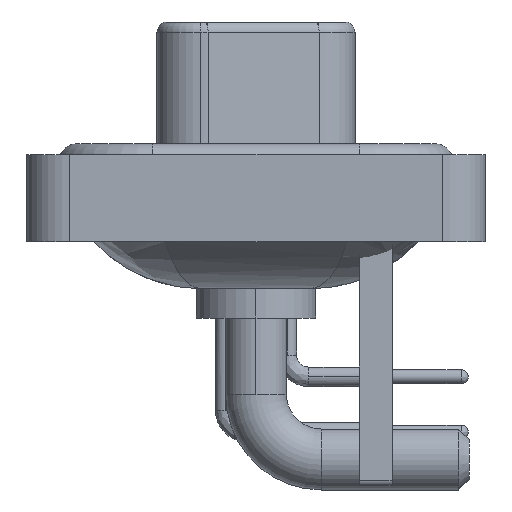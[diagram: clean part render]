
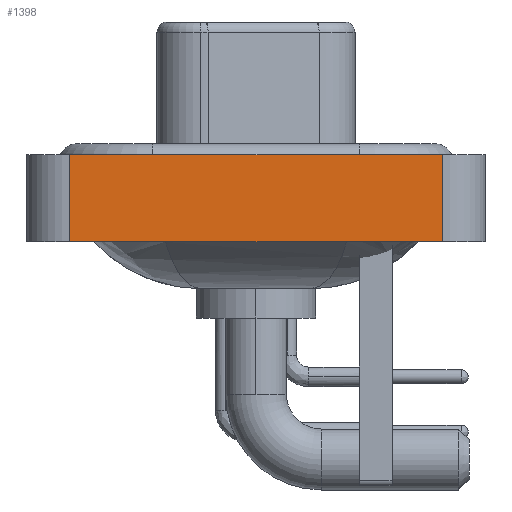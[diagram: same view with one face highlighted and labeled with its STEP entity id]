
A CAD part, left-side view. The second image highlights one B-rep face of the part: STEP entity #1398.
In plain terms, the highlighted planar face has unit normal (-1, 0, 0).
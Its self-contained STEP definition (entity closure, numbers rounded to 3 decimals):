
#428 = PLANE ( 'NONE',  #26858 ) ;
#519 = CARTESIAN_POINT ( 'NONE',  ( -7.35, 8.55, -3.6 ) ) ;
#929 = CARTESIAN_POINT ( 'NONE',  ( -7.35, 8.55, -3.6 ) ) ;
#1398 = ADVANCED_FACE ( 'NONE', ( #18277 ), #428, .T. ) ;
#2230 = EDGE_CURVE ( 'NONE', #17296, #16512, #19049, .T. ) ;
#3063 = DIRECTION ( 'NONE',  ( -1., 0., 0. ) ) ;
#4238 = CARTESIAN_POINT ( 'NONE',  ( -7.35, 8.55, 0.4 ) ) ;
#6524 = VECTOR ( 'NONE', #18590, 1000. ) ;
#7141 = VECTOR ( 'NONE', #9391, 1000. ) ;
#9391 = DIRECTION ( 'NONE',  ( 0., 0., 1. ) ) ;
#9456 = CARTESIAN_POINT ( 'NONE',  ( -7.35, -8.55, -3.6 ) ) ;
#9499 = LINE ( 'NONE', #13789, #28055 ) ;
#9691 = CARTESIAN_POINT ( 'NONE',  ( -7.35, -8.55, 0.4 ) ) ;
#10008 = EDGE_LOOP ( 'NONE', ( #10901, #12524, #17019, #13452 ) ) ;
#10021 = CARTESIAN_POINT ( 'NONE',  ( -7.35, -8.55, -3.6 ) ) ;
#10263 = EDGE_CURVE ( 'NONE', #16512, #11196, #16607, .T. ) ;
#10901 = ORIENTED_EDGE ( 'NONE', *, *, #28293, .T. ) ;
#11196 = VERTEX_POINT ( 'NONE', #13530 ) ;
#12195 = VECTOR ( 'NONE', #23393, 1000. ) ;
#12524 = ORIENTED_EDGE ( 'NONE', *, *, #10263, .F. ) ;
#13452 = ORIENTED_EDGE ( 'NONE', *, *, #19884, .T. ) ;
#13530 = CARTESIAN_POINT ( 'NONE',  ( -7.35, -8.55, 0.4 ) ) ;
#13789 = CARTESIAN_POINT ( 'NONE',  ( -7.35, -8.55, -3.6 ) ) ;
#16512 = VERTEX_POINT ( 'NONE', #4238 ) ;
#16607 = LINE ( 'NONE', #9691, #12195 ) ;
#17019 = ORIENTED_EDGE ( 'NONE', *, *, #2230, .F. ) ;
#17296 = VERTEX_POINT ( 'NONE', #929 ) ;
#18277 = FACE_OUTER_BOUND ( 'NONE', #10008, .T. ) ;
#18482 = DIRECTION ( 'NONE',  ( 0., 0., 1. ) ) ;
#18590 = DIRECTION ( 'NONE',  ( 0., -1., 0. ) ) ;
#19049 = LINE ( 'NONE', #519, #7141 ) ;
#19884 = EDGE_CURVE ( 'NONE', #17296, #20099, #27732, .T. ) ;
#20099 = VERTEX_POINT ( 'NONE', #10021 ) ;
#23122 = DIRECTION ( 'NONE',  ( 0., 0., 1. ) ) ;
#23264 = CARTESIAN_POINT ( 'NONE',  ( -7.35, -8.55, -3.6 ) ) ;
#23393 = DIRECTION ( 'NONE',  ( 0., -1., 0. ) ) ;
#26858 = AXIS2_PLACEMENT_3D ( 'NONE', #23264, #3063, #23122 ) ;
#27732 = LINE ( 'NONE', #9456, #6524 ) ;
#28055 = VECTOR ( 'NONE', #18482, 1000. ) ;
#28293 = EDGE_CURVE ( 'NONE', #20099, #11196, #9499, .T. ) ;
